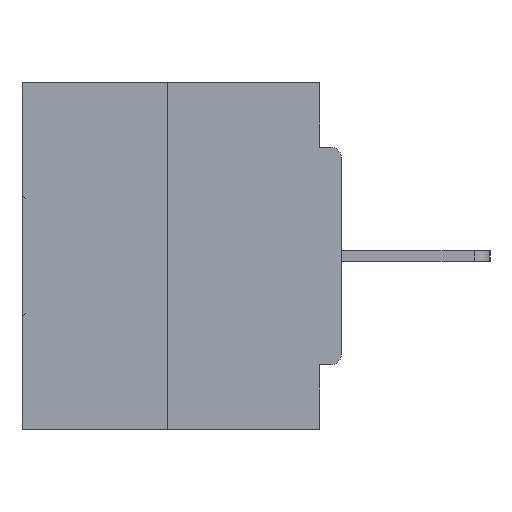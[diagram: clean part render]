
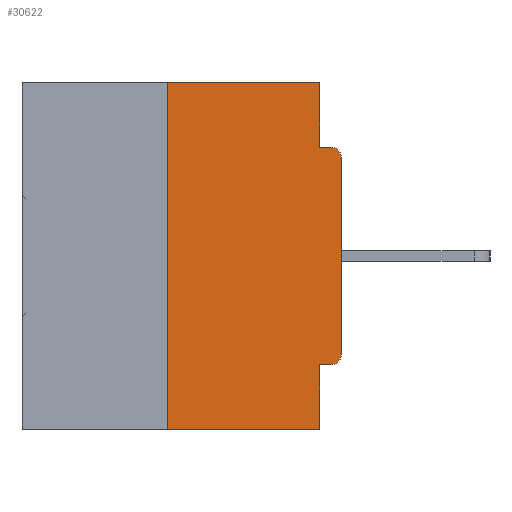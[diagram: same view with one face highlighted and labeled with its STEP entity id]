
A CAD part, left-side view. The second image highlights one B-rep face of the part: STEP entity #30622.
In plain terms, the highlighted planar face has unit normal (-1, 0, 0).
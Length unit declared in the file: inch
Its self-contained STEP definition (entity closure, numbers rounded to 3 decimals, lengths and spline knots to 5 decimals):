
#121 = LINE ( 'NONE', #19854, #34002 ) ;
#480 = CARTESIAN_POINT ( 'NONE',  ( 0., 0.46, 0. ) ) ;
#798 = DIRECTION ( 'NONE',  ( -1., 0., 0. ) ) ;
#1409 = VECTOR ( 'NONE', #16680, 39.37008 ) ;
#1595 = PLANE ( 'NONE',  #26349 ) ;
#1844 = LINE ( 'NONE', #36041, #9200 ) ;
#2964 = LINE ( 'NONE', #17981, #10506 ) ;
#2975 = DIRECTION ( 'NONE',  ( 0., 0., -1. ) ) ;
#3339 = CARTESIAN_POINT ( 'NONE',  ( 0., 0.015, -0.1085 ) ) ;
#4230 = ORIENTED_EDGE ( 'NONE', *, *, #18215, .F. ) ;
#4396 = CARTESIAN_POINT ( 'NONE',  ( 0., 0.25, -0.5 ) ) ;
#4649 = AXIS2_PLACEMENT_3D ( 'NONE', #26148, #798, #15230 ) ;
#5242 = CARTESIAN_POINT ( 'NONE',  ( 0., 0.25, 0. ) ) ;
#5408 = CARTESIAN_POINT ( 'NONE',  ( 0., 0.031, -0.5 ) ) ;
#6067 = EDGE_CURVE ( 'NONE', #14041, #31021, #20074, .T. ) ;
#6350 = EDGE_CURVE ( 'NONE', #33194, #25595, #15260, .T. ) ;
#7218 = CARTESIAN_POINT ( 'NONE',  ( 0., 0.031, -0.5 ) ) ;
#7578 = ORIENTED_EDGE ( 'NONE', *, *, #18299, .T. ) ;
#9200 = VECTOR ( 'NONE', #24772, 39.37008 ) ;
#10506 = VECTOR ( 'NONE', #26068, 39.37008 ) ;
#10872 = LINE ( 'NONE', #19151, #12061 ) ;
#12061 = VECTOR ( 'NONE', #19335, 39.37008 ) ;
#12490 = CARTESIAN_POINT ( 'NONE',  ( 0., 0.46, 0. ) ) ;
#12729 = LINE ( 'NONE', #29671, #12755 ) ;
#12755 = VECTOR ( 'NONE', #15373, 39.37008 ) ;
#13036 = DIRECTION ( 'NONE',  ( 1., 0., 0. ) ) ;
#13051 = CARTESIAN_POINT ( 'NONE',  ( 0., 0.031, -0.4065 ) ) ;
#14041 = VERTEX_POINT ( 'NONE', #24035 ) ;
#14536 = VERTEX_POINT ( 'NONE', #35850 ) ;
#14878 = VERTEX_POINT ( 'NONE', #13051 ) ;
#15230 = DIRECTION ( 'NONE',  ( 0., 0., -1. ) ) ;
#15235 = ORIENTED_EDGE ( 'NONE', *, *, #34086, .F. ) ;
#15260 = CIRCLE ( 'NONE', #16465, 0.015 ) ;
#15373 = DIRECTION ( 'NONE',  ( 0., 0., 1. ) ) ;
#15673 = DIRECTION ( 'NONE',  ( 0., 0., -1. ) ) ;
#16319 = CARTESIAN_POINT ( 'NONE',  ( 0., 0.031, -0.0935 ) ) ;
#16465 = AXIS2_PLACEMENT_3D ( 'NONE', #3339, #20641, #2975 ) ;
#16680 = DIRECTION ( 'NONE',  ( 0., 0., -1. ) ) ;
#17021 = DIRECTION ( 'NONE',  ( 0., 0., 1. ) ) ;
#17306 = ORIENTED_EDGE ( 'NONE', *, *, #6350, .T. ) ;
#17426 = CARTESIAN_POINT ( 'NONE',  ( 0., 0.031, 0. ) ) ;
#17981 = CARTESIAN_POINT ( 'NONE',  ( 0., 0., -0.4065 ) ) ;
#18215 = EDGE_CURVE ( 'NONE', #34986, #30145, #12729, .T. ) ;
#18299 = EDGE_CURVE ( 'NONE', #34986, #29359, #1844, .T. ) ;
#18363 = EDGE_CURVE ( 'NONE', #14878, #29359, #19877, .T. ) ;
#19138 = VECTOR ( 'NONE', #28892, 39.37008 ) ;
#19151 = CARTESIAN_POINT ( 'NONE',  ( 0., 0., -0.0935 ) ) ;
#19335 = DIRECTION ( 'NONE',  ( 0., -1., 0. ) ) ;
#19854 = CARTESIAN_POINT ( 'NONE',  ( 0., 0., 0. ) ) ;
#19877 = LINE ( 'NONE', #5408, #1409 ) ;
#20074 = LINE ( 'NONE', #17426, #19138 ) ;
#20641 = DIRECTION ( 'NONE',  ( -1., 0., 0. ) ) ;
#20878 = CIRCLE ( 'NONE', #4649, 0.015 ) ;
#22241 = CARTESIAN_POINT ( 'NONE',  ( 0., 0.015, -0.0935 ) ) ;
#22390 = EDGE_CURVE ( 'NONE', #30145, #14041, #35214, .T. ) ;
#22813 = EDGE_CURVE ( 'NONE', #28270, #14536, #20878, .T. ) ;
#24035 = CARTESIAN_POINT ( 'NONE',  ( 0., 0.031, 0. ) ) ;
#24772 = DIRECTION ( 'NONE',  ( 0., -1., 0. ) ) ;
#24978 = EDGE_CURVE ( 'NONE', #28270, #14878, #2964, .T. ) ;
#25595 = VERTEX_POINT ( 'NONE', #22241 ) ;
#26068 = DIRECTION ( 'NONE',  ( 0., 1., 0. ) ) ;
#26148 = CARTESIAN_POINT ( 'NONE',  ( 0., 0.015, -0.3915 ) ) ;
#26349 = AXIS2_PLACEMENT_3D ( 'NONE', #12490, #13036, #15673 ) ;
#27111 = EDGE_LOOP ( 'NONE', ( #34656, #4230, #7578, #33740, #32183, #35360, #28362, #17306, #15235, #32070 ) ) ;
#27341 = FACE_OUTER_BOUND ( 'NONE', #27111, .T. ) ;
#27755 = EDGE_CURVE ( 'NONE', #14536, #33194, #121, .T. ) ;
#28270 = VERTEX_POINT ( 'NONE', #33901 ) ;
#28362 = ORIENTED_EDGE ( 'NONE', *, *, #27755, .T. ) ;
#28892 = DIRECTION ( 'NONE',  ( 0., 0., -1. ) ) ;
#29359 = VERTEX_POINT ( 'NONE', #7218 ) ;
#29399 = DIRECTION ( 'NONE',  ( 0., -1., 0. ) ) ;
#29671 = CARTESIAN_POINT ( 'NONE',  ( 0., 0.25, 0. ) ) ;
#30145 = VERTEX_POINT ( 'NONE', #5242 ) ;
#30622 = ADVANCED_FACE ( 'NONE', ( #27341 ), #1595, .F. ) ;
#31021 = VERTEX_POINT ( 'NONE', #16319 ) ;
#31041 = VECTOR ( 'NONE', #29399, 39.37008 ) ;
#32070 = ORIENTED_EDGE ( 'NONE', *, *, #6067, .F. ) ;
#32183 = ORIENTED_EDGE ( 'NONE', *, *, #24978, .F. ) ;
#33194 = VERTEX_POINT ( 'NONE', #35986 ) ;
#33740 = ORIENTED_EDGE ( 'NONE', *, *, #18363, .F. ) ;
#33901 = CARTESIAN_POINT ( 'NONE',  ( 0., 0.015, -0.4065 ) ) ;
#34002 = VECTOR ( 'NONE', #17021, 39.37008 ) ;
#34086 = EDGE_CURVE ( 'NONE', #31021, #25595, #10872, .T. ) ;
#34656 = ORIENTED_EDGE ( 'NONE', *, *, #22390, .F. ) ;
#34986 = VERTEX_POINT ( 'NONE', #4396 ) ;
#35214 = LINE ( 'NONE', #480, #31041 ) ;
#35360 = ORIENTED_EDGE ( 'NONE', *, *, #22813, .T. ) ;
#35850 = CARTESIAN_POINT ( 'NONE',  ( 0., 0., -0.3915 ) ) ;
#35986 = CARTESIAN_POINT ( 'NONE',  ( 0., 0., -0.1085 ) ) ;
#36041 = CARTESIAN_POINT ( 'NONE',  ( 0., 0.46, -0.5 ) ) ;
